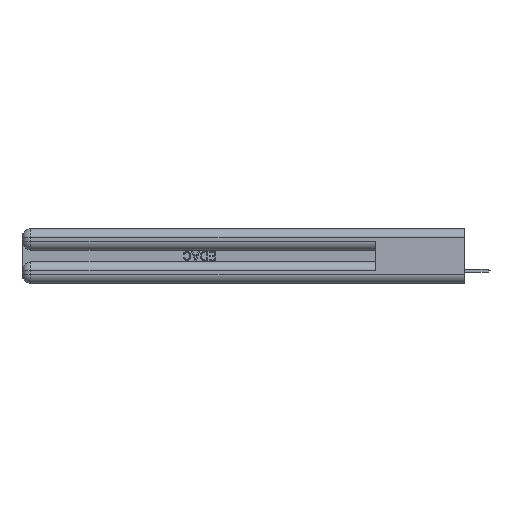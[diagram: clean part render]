
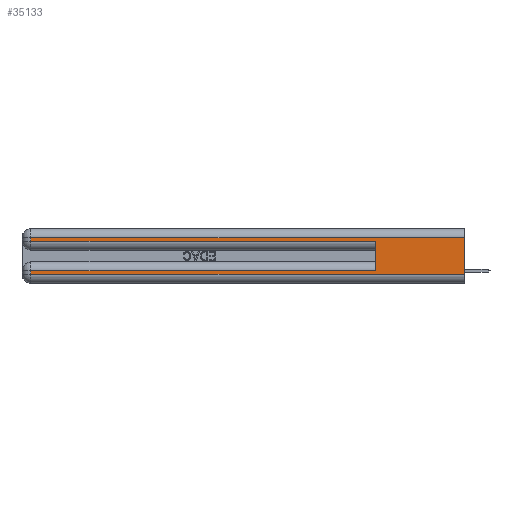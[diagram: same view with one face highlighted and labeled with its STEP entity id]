
A CAD part, left-side view. The second image highlights one B-rep face of the part: STEP entity #35133.
In plain terms, the highlighted planar face has unit normal (-1, 0, 0).
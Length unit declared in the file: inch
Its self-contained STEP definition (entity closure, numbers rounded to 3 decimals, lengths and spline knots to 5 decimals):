
#717 = EDGE_CURVE ( 'NONE', #30744, #6547, #18463, .T. ) ;
#1338 = DIRECTION ( 'NONE',  ( 0., 0., -1. ) ) ;
#1858 = VECTOR ( 'NONE', #23755, 39.37008 ) ;
#2268 = EDGE_CURVE ( 'NONE', #4949, #33232, #15856, .T. ) ;
#3102 = DIRECTION ( 'NONE',  ( 0., 0., -1. ) ) ;
#3202 = CARTESIAN_POINT ( 'NONE',  ( 0., 0., 0.085 ) ) ;
#3283 = DIRECTION ( 'NONE',  ( 0., 1., 0. ) ) ;
#4249 = VERTEX_POINT ( 'NONE', #16830 ) ;
#4556 = CARTESIAN_POINT ( 'NONE',  ( 0., 2.94, 0.31 ) ) ;
#4949 = VERTEX_POINT ( 'NONE', #8616 ) ;
#5990 = ORIENTED_EDGE ( 'NONE', *, *, #7862, .F. ) ;
#6547 = VERTEX_POINT ( 'NONE', #9400 ) ;
#6696 = LINE ( 'NONE', #35567, #10058 ) ;
#7862 = EDGE_CURVE ( 'NONE', #4949, #19071, #32737, .T. ) ;
#8121 = VECTOR ( 'NONE', #3283, 39.37008 ) ;
#8275 = VECTOR ( 'NONE', #3102, 39.37008 ) ;
#8616 = CARTESIAN_POINT ( 'NONE',  ( 0., 0., 0.31 ) ) ;
#9400 = CARTESIAN_POINT ( 'NONE',  ( 0., 2.94, 0.06 ) ) ;
#10058 = VECTOR ( 'NONE', #17092, 39.37008 ) ;
#11302 = VERTEX_POINT ( 'NONE', #22222 ) ;
#11358 = CARTESIAN_POINT ( 'NONE',  ( 0., 0., 0.37 ) ) ;
#11372 = EDGE_CURVE ( 'NONE', #11302, #4249, #6696, .T. ) ;
#12144 = EDGE_CURVE ( 'NONE', #6547, #19071, #14446, .T. ) ;
#12590 = ORIENTED_EDGE ( 'NONE', *, *, #2268, .T. ) ;
#13674 = ORIENTED_EDGE ( 'NONE', *, *, #12144, .T. ) ;
#14142 = VECTOR ( 'NONE', #17419, 39.37008 ) ;
#14151 = CARTESIAN_POINT ( 'NONE',  ( 0., 0., 0.06 ) ) ;
#14416 = CARTESIAN_POINT ( 'NONE',  ( 0., 0., 0.285 ) ) ;
#14446 = LINE ( 'NONE', #14151, #1858 ) ;
#14544 = EDGE_LOOP ( 'NONE', ( #5990, #12590, #31435, #15440, #29473, #15465, #20005, #13674 ) ) ;
#14685 = CARTESIAN_POINT ( 'NONE',  ( 0., 2.94, 0.085 ) ) ;
#14919 = VERTEX_POINT ( 'NONE', #26292 ) ;
#14960 = DIRECTION ( 'NONE',  ( 0., 0., -1. ) ) ;
#15440 = ORIENTED_EDGE ( 'NONE', *, *, #35562, .T. ) ;
#15465 = ORIENTED_EDGE ( 'NONE', *, *, #33666, .T. ) ;
#15856 = LINE ( 'NONE', #34064, #8121 ) ;
#16830 = CARTESIAN_POINT ( 'NONE',  ( 0., 0.6, 0.285 ) ) ;
#17092 = DIRECTION ( 'NONE',  ( 0., 0., 1. ) ) ;
#17190 = DIRECTION ( 'NONE',  ( 1., 0., 0. ) ) ;
#17419 = DIRECTION ( 'NONE',  ( 0., -1., 0. ) ) ;
#18463 = LINE ( 'NONE', #36626, #8275 ) ;
#19071 = VERTEX_POINT ( 'NONE', #35876 ) ;
#19922 = CARTESIAN_POINT ( 'NONE',  ( 0., 2.94, 0.37 ) ) ;
#20005 = ORIENTED_EDGE ( 'NONE', *, *, #717, .T. ) ;
#20478 = AXIS2_PLACEMENT_3D ( 'NONE', #11358, #17190, #23811 ) ;
#20599 = PLANE ( 'NONE',  #20478 ) ;
#21583 = VECTOR ( 'NONE', #27881, 39.37008 ) ;
#22222 = CARTESIAN_POINT ( 'NONE',  ( 0., 0.6, 0.085 ) ) ;
#23145 = VECTOR ( 'NONE', #14960, 39.37008 ) ;
#23755 = DIRECTION ( 'NONE',  ( 0., -1., 0. ) ) ;
#23811 = DIRECTION ( 'NONE',  ( 0., 0., -1. ) ) ;
#23850 = LINE ( 'NONE', #14416, #14142 ) ;
#26292 = CARTESIAN_POINT ( 'NONE',  ( 0., 2.94, 0.285 ) ) ;
#26753 = FACE_OUTER_BOUND ( 'NONE', #14544, .T. ) ;
#26805 = LINE ( 'NONE', #19922, #28152 ) ;
#27473 = CARTESIAN_POINT ( 'NONE',  ( 0., 0., 0.37 ) ) ;
#27881 = DIRECTION ( 'NONE',  ( 0., 1., 0. ) ) ;
#28152 = VECTOR ( 'NONE', #1338, 39.37008 ) ;
#29473 = ORIENTED_EDGE ( 'NONE', *, *, #11372, .F. ) ;
#29720 = LINE ( 'NONE', #3202, #21583 ) ;
#30744 = VERTEX_POINT ( 'NONE', #14685 ) ;
#31435 = ORIENTED_EDGE ( 'NONE', *, *, #36123, .T. ) ;
#32737 = LINE ( 'NONE', #27473, #23145 ) ;
#33232 = VERTEX_POINT ( 'NONE', #4556 ) ;
#33666 = EDGE_CURVE ( 'NONE', #11302, #30744, #29720, .T. ) ;
#34064 = CARTESIAN_POINT ( 'NONE',  ( 0., 0., 0.31 ) ) ;
#35133 = ADVANCED_FACE ( 'NONE', ( #26753 ), #20599, .F. ) ;
#35562 = EDGE_CURVE ( 'NONE', #14919, #4249, #23850, .T. ) ;
#35567 = CARTESIAN_POINT ( 'NONE',  ( 0., 0.6, 0.145 ) ) ;
#35876 = CARTESIAN_POINT ( 'NONE',  ( 0., 0., 0.06 ) ) ;
#36123 = EDGE_CURVE ( 'NONE', #33232, #14919, #26805, .T. ) ;
#36626 = CARTESIAN_POINT ( 'NONE',  ( 0., 2.94, 0.37 ) ) ;
